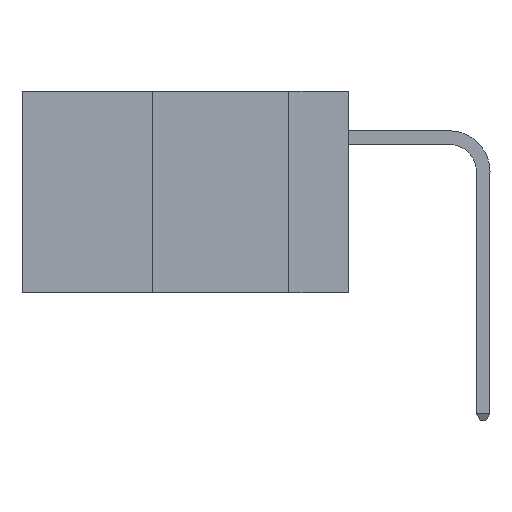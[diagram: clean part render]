
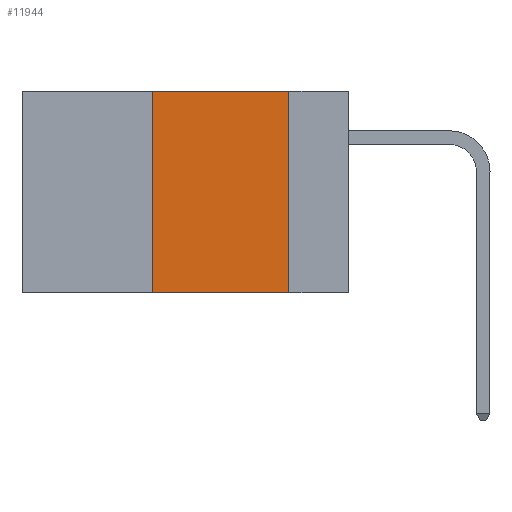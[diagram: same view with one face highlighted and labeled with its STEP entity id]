
A CAD part, left-side view. The second image highlights one B-rep face of the part: STEP entity #11944.
In plain terms, the highlighted planar face has unit normal (-1, 0, 0).
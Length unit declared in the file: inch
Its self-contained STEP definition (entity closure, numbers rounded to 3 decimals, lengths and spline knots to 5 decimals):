
#351 = CARTESIAN_POINT ( 'NONE',  ( 0., 0.6, 0. ) ) ;
#376 = DIRECTION ( 'NONE',  ( 0., 0., -1. ) ) ;
#1324 = CARTESIAN_POINT ( 'NONE',  ( 0., 0.11, 0. ) ) ;
#2207 = DIRECTION ( 'NONE',  ( 1., 0., 0. ) ) ;
#2543 = CARTESIAN_POINT ( 'NONE',  ( 0., 0.36, -0.37 ) ) ;
#3172 = DIRECTION ( 'NONE',  ( 0., -1., 0. ) ) ;
#3881 = LINE ( 'NONE', #7878, #8276 ) ;
#4847 = EDGE_CURVE ( 'NONE', #13913, #14377, #5263, .T. ) ;
#5263 = LINE ( 'NONE', #8982, #9613 ) ;
#6046 = LINE ( 'NONE', #21684, #11544 ) ;
#6246 = VERTEX_POINT ( 'NONE', #1324 ) ;
#7878 = CARTESIAN_POINT ( 'NONE',  ( 0., 0.11, 0. ) ) ;
#8212 = AXIS2_PLACEMENT_3D ( 'NONE', #351, #2207, #15093 ) ;
#8276 = VECTOR ( 'NONE', #376, 39.37008 ) ;
#8764 = CARTESIAN_POINT ( 'NONE',  ( 0., 0.11, -0.37 ) ) ;
#8982 = CARTESIAN_POINT ( 'NONE',  ( 0., 0.36, 0. ) ) ;
#9613 = VECTOR ( 'NONE', #19882, 39.37008 ) ;
#9804 = EDGE_CURVE ( 'NONE', #6246, #22353, #3881, .T. ) ;
#10828 = DIRECTION ( 'NONE',  ( 0., -1., 0. ) ) ;
#11290 = EDGE_CURVE ( 'NONE', #14377, #6246, #13914, .T. ) ;
#11395 = CARTESIAN_POINT ( 'NONE',  ( 0., 0.36, 0. ) ) ;
#11457 = PLANE ( 'NONE',  #8212 ) ;
#11544 = VECTOR ( 'NONE', #10828, 39.37008 ) ;
#11944 = ADVANCED_FACE ( 'NONE', ( #18988 ), #11457, .F. ) ;
#12707 = EDGE_LOOP ( 'NONE', ( #23344, #21386, #22499, #19404 ) ) ;
#13913 = VERTEX_POINT ( 'NONE', #2543 ) ;
#13914 = LINE ( 'NONE', #14219, #23558 ) ;
#14219 = CARTESIAN_POINT ( 'NONE',  ( 0., 0.6, 0. ) ) ;
#14377 = VERTEX_POINT ( 'NONE', #11395 ) ;
#15093 = DIRECTION ( 'NONE',  ( 0., 0., -1. ) ) ;
#18988 = FACE_OUTER_BOUND ( 'NONE', #12707, .T. ) ;
#19404 = ORIENTED_EDGE ( 'NONE', *, *, #20554, .T. ) ;
#19882 = DIRECTION ( 'NONE',  ( 0., 0., 1. ) ) ;
#20554 = EDGE_CURVE ( 'NONE', #13913, #22353, #6046, .T. ) ;
#21386 = ORIENTED_EDGE ( 'NONE', *, *, #11290, .F. ) ;
#21684 = CARTESIAN_POINT ( 'NONE',  ( 0., 0.6, -0.37 ) ) ;
#22353 = VERTEX_POINT ( 'NONE', #8764 ) ;
#22499 = ORIENTED_EDGE ( 'NONE', *, *, #4847, .F. ) ;
#23344 = ORIENTED_EDGE ( 'NONE', *, *, #9804, .F. ) ;
#23558 = VECTOR ( 'NONE', #3172, 39.37008 ) ;
